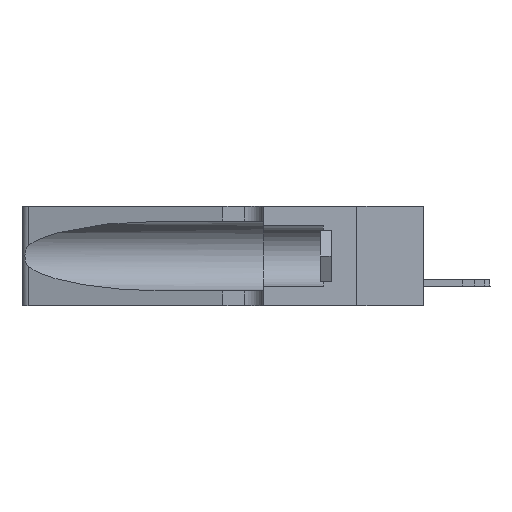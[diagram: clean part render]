
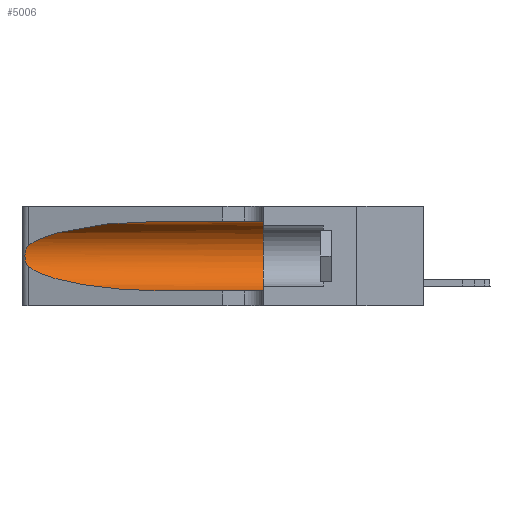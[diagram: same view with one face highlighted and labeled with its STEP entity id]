
A CAD part, left-side view. The second image highlights one B-rep face of the part: STEP entity #5006.
In plain terms, the highlighted cylindrical face has radius 3.308 mm (diameter 6.617 mm), a partial arc.
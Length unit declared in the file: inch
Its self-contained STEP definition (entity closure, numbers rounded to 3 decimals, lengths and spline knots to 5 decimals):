
#21 = DIRECTION ( 'NONE',  ( 0., -1., 0. ) ) ;
#253 = CYLINDRICAL_SURFACE ( 'NONE', #3704, 0.13025 ) ;
#1270 = VERTEX_POINT ( 'NONE', #9371 ) ;
#1342 = EDGE_CURVE ( 'NONE', #15736, #1270, #16693, .T. ) ;
#1683 = CARTESIAN_POINT ( 'NONE',  ( 0.18966, 0.96281, 0.05475 ) ) ;
#1715 = CARTESIAN_POINT ( 'NONE',  ( 0.25639, 1.23186, 0.15144 ) ) ;
#1873 = CARTESIAN_POINT ( 'NONE',  ( 0.25555, 1.22993, 0.14849 ) ) ;
#2886 = EDGE_CURVE ( 'NONE', #8563, #23631, #16329, .T. ) ;
#3217 = ORIENTED_EDGE ( 'NONE', *, *, #12619, .T. ) ;
#3377 = ORIENTED_EDGE ( 'NONE', *, *, #2886, .T. ) ;
#3617 = DIRECTION ( 'NONE',  ( 0., -1., 0. ) ) ;
#3688 = AXIS2_PLACEMENT_3D ( 'NONE', #7895, #7814, #7598 ) ;
#3704 = AXIS2_PLACEMENT_3D ( 'NONE', #17009, #21, #5525 ) ;
#3761 = CIRCLE ( 'NONE', #3688, 0.13025 ) ;
#3905 = CARTESIAN_POINT ( 'NONE',  ( 0.25487, 1.22718, 0.14631 ) ) ;
#4726 = CARTESIAN_POINT ( 'NONE',  ( 0.1305, 1.61858, 0.31525 ) ) ;
#4921 = EDGE_CURVE ( 'NONE', #11477, #8563, #10438, .T. ) ;
#5006 = ADVANCED_FACE ( 'NONE', ( #21504 ), #253, .F. ) ;
#5350 = CARTESIAN_POINT ( 'NONE',  ( 0.25487, 1.22718, 0.14631 ) ) ;
#5379 = CARTESIAN_POINT ( 'NONE',  ( 0.25555, 1.22994, 0.2215 ) ) ;
#5525 = DIRECTION ( 'NONE',  ( 0., 0., -1. ) ) ;
#6006 =( BOUNDED_CURVE ( )  B_SPLINE_CURVE ( 3, ( #5350, #22276, #1683, #12953 ),
 .UNSPECIFIED., .F., .F. ) 
 B_SPLINE_CURVE_WITH_KNOTS ( ( 4, 4 ),
 ( 3.44316, 4.71239 ),
 .UNSPECIFIED. ) 
 CURVE ( )  GEOMETRIC_REPRESENTATION_ITEM ( )  RATIONAL_B_SPLINE_CURVE ( ( 1., 0.87, 0.87, 1. ) ) 
 REPRESENTATION_ITEM ( '' )  );
#6429 = CARTESIAN_POINT ( 'NONE',  ( 0.25487, 1.22718, 0.22369 ) ) ;
#7199 = LINE ( 'NONE', #4726, #23131 ) ;
#7361 = CARTESIAN_POINT ( 'NONE',  ( 0.25639, 1.23184, 0.21858 ) ) ;
#7365 = CARTESIAN_POINT ( 'NONE',  ( 0.1305, 0.72297, 0.05475 ) ) ;
#7598 = DIRECTION ( 'NONE',  ( 0., 0., 1. ) ) ;
#7814 = DIRECTION ( 'NONE',  ( 0., 1., 0. ) ) ;
#7851 = EDGE_CURVE ( 'NONE', #11477, #19105, #7199, .T. ) ;
#7895 = CARTESIAN_POINT ( 'NONE',  ( 0.1305, 0.35, 0.185 ) ) ;
#8225 = ORIENTED_EDGE ( 'NONE', *, *, #20338, .F. ) ;
#8563 = VERTEX_POINT ( 'NONE', #6429 ) ;
#9346 = CARTESIAN_POINT ( 'NONE',  ( 0.25854, 1.2359, 0.20912 ) ) ;
#9371 = CARTESIAN_POINT ( 'NONE',  ( 0.1305, 0.35, 0.05475 ) ) ;
#9432 = CARTESIAN_POINT ( 'NONE',  ( 0.26018, 1.23835, 0.19895 ) ) ;
#9495 = CARTESIAN_POINT ( 'NONE',  ( 0.18966, 0.96281, 0.31525 ) ) ;
#9571 = CARTESIAN_POINT ( 'NONE',  ( 0.1305, 0.72297, 0.31525 ) ) ;
#9595 = ORIENTED_EDGE ( 'NONE', *, *, #1342, .T. ) ;
#10438 =( BOUNDED_CURVE ( )  B_SPLINE_CURVE ( 3, ( #9571, #9495, #20817, #11415 ),
 .UNSPECIFIED., .F., .F. ) 
 B_SPLINE_CURVE_WITH_KNOTS ( ( 4, 4 ),
 ( 1.5708, 2.84003 ),
 .UNSPECIFIED. ) 
 CURVE ( )  GEOMETRIC_REPRESENTATION_ITEM ( )  RATIONAL_B_SPLINE_CURVE ( ( 1., 0.87, 0.87, 1. ) ) 
 REPRESENTATION_ITEM ( '' )  );
#11193 = CARTESIAN_POINT ( 'NONE',  ( 0.25856, 1.23593, 0.16098 ) ) ;
#11415 = CARTESIAN_POINT ( 'NONE',  ( 0.25487, 1.22718, 0.22369 ) ) ;
#11477 = VERTEX_POINT ( 'NONE', #15001 ) ;
#11584 = CARTESIAN_POINT ( 'NONE',  ( 0.1305, 0.35, 0.31525 ) ) ;
#12619 = EDGE_CURVE ( 'NONE', #23631, #15736, #6006, .T. ) ;
#12953 = CARTESIAN_POINT ( 'NONE',  ( 0.1305, 0.72297, 0.05475 ) ) ;
#12980 = CARTESIAN_POINT ( 'NONE',  ( 0.25789, 1.23486, 0.15765 ) ) ;
#14376 = ORIENTED_EDGE ( 'NONE', *, *, #7851, .F. ) ;
#14911 = CARTESIAN_POINT ( 'NONE',  ( 0.1305, 1.61858, 0.05475 ) ) ;
#15001 = CARTESIAN_POINT ( 'NONE',  ( 0.1305, 0.72297, 0.31525 ) ) ;
#15736 = VERTEX_POINT ( 'NONE', #7365 ) ;
#16329 = B_SPLINE_CURVE_WITH_KNOTS ( 'NONE', 3,
 ( #18850, #5379, #7361, #20583, #9346, #9432, #24270, #22467, #22632, #11193, #12980, #1715, #1873, #18679 ),
 .UNSPECIFIED., .F., .F.,
 ( 4, 2, 2, 2, 2, 2, 4 ),
 ( 0., 0.00027, 0.00053, 0.00107, 0.0016, 0.00187, 0.00214 ),
 .UNSPECIFIED. ) ;
#16693 = LINE ( 'NONE', #14911, #20256 ) ;
#17009 = CARTESIAN_POINT ( 'NONE',  ( 0.1305, 1.61858, 0.185 ) ) ;
#18679 = CARTESIAN_POINT ( 'NONE',  ( 0.25487, 1.22718, 0.14631 ) ) ;
#18850 = CARTESIAN_POINT ( 'NONE',  ( 0.25487, 1.22718, 0.22369 ) ) ;
#19105 = VERTEX_POINT ( 'NONE', #11584 ) ;
#19711 = EDGE_LOOP ( 'NONE', ( #21341, #3377, #3217, #9595, #8225, #14376 ) ) ;
#20256 = VECTOR ( 'NONE', #3617, 39.37008 ) ;
#20338 = EDGE_CURVE ( 'NONE', #19105, #1270, #3761, .T. ) ;
#20583 = CARTESIAN_POINT ( 'NONE',  ( 0.25787, 1.23484, 0.2124 ) ) ;
#20817 = CARTESIAN_POINT ( 'NONE',  ( 0.2373, 1.15595, 0.28018 ) ) ;
#21341 = ORIENTED_EDGE ( 'NONE', *, *, #4921, .T. ) ;
#21504 = FACE_OUTER_BOUND ( 'NONE', #19711, .T. ) ;
#22276 = CARTESIAN_POINT ( 'NONE',  ( 0.2373, 1.15595, 0.08982 ) ) ;
#22467 = CARTESIAN_POINT ( 'NONE',  ( 0.26075, 1.23896, 0.178 ) ) ;
#22632 = CARTESIAN_POINT ( 'NONE',  ( 0.26017, 1.23833, 0.17102 ) ) ;
#23131 = VECTOR ( 'NONE', #23545, 39.37008 ) ;
#23545 = DIRECTION ( 'NONE',  ( 0., -1., 0. ) ) ;
#23631 = VERTEX_POINT ( 'NONE', #3905 ) ;
#24270 = CARTESIAN_POINT ( 'NONE',  ( 0.26075, 1.23896, 0.19203 ) ) ;
